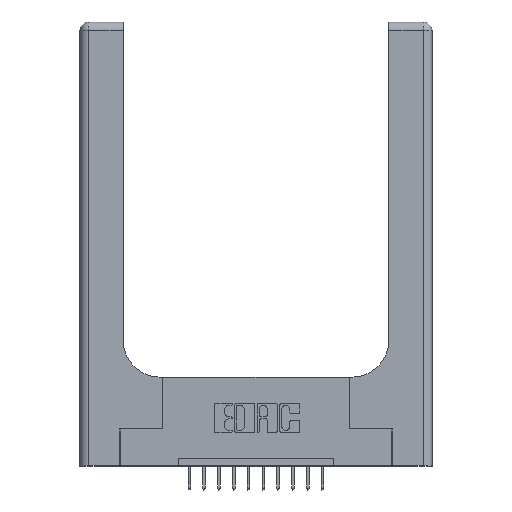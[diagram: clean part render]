
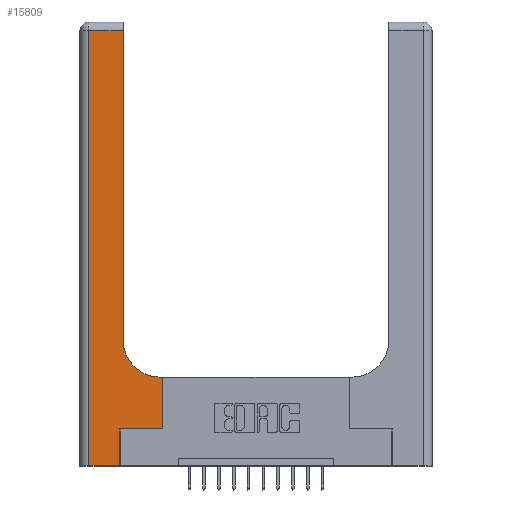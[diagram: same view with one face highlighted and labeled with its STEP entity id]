
A CAD part, top view. The second image highlights one B-rep face of the part: STEP entity #15809.
In plain terms, the highlighted planar face has unit normal (0, 0, 1).
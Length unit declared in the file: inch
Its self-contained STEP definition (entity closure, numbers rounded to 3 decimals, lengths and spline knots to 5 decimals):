
#538 = EDGE_CURVE ( 'NONE', #6167, #1486, #4916, .T. ) ;
#605 = CARTESIAN_POINT ( 'NONE',  ( 0.5585, 0.25, 0.37 ) ) ;
#1486 = VERTEX_POINT ( 'NONE', #4777 ) ;
#1551 = CARTESIAN_POINT ( 'NONE',  ( 0.2915, 0.85, 0.37 ) ) ;
#1597 = LINE ( 'NONE', #6322, #7417 ) ;
#1854 = CARTESIAN_POINT ( 'NONE',  ( 0.2915, 2.94, 0.37 ) ) ;
#2332 = ORIENTED_EDGE ( 'NONE', *, *, #2520, .T. ) ;
#2349 = EDGE_CURVE ( 'NONE', #9811, #10338, #3367, .T. ) ;
#2389 = AXIS2_PLACEMENT_3D ( 'NONE', #6946, #14669, #8240 ) ;
#2520 = EDGE_CURVE ( 'NONE', #7025, #6167, #9157, .T. ) ;
#2974 = LINE ( 'NONE', #16132, #4400 ) ;
#3108 = DIRECTION ( 'NONE',  ( 0., 1., 0. ) ) ;
#3366 = LINE ( 'NONE', #6575, #16765 ) ;
#3367 = LINE ( 'NONE', #4413, #13280 ) ;
#3517 = DIRECTION ( 'NONE',  ( -1., 0., 0. ) ) ;
#3970 = ORIENTED_EDGE ( 'NONE', *, *, #5538, .T. ) ;
#4192 = DIRECTION ( 'NONE',  ( 0., 1., 0. ) ) ;
#4400 = VECTOR ( 'NONE', #16188, 39.37008 ) ;
#4413 = CARTESIAN_POINT ( 'NONE',  ( 0.2915, 3., 0.37 ) ) ;
#4546 = EDGE_LOOP ( 'NONE', ( #6118, #3970, #15986, #16181, #9158, #2332, #13299, #15237, #9519 ) ) ;
#4726 = VECTOR ( 'NONE', #15350, 39.37008 ) ;
#4777 = CARTESIAN_POINT ( 'NONE',  ( 0.5585, 0.6, 0.37 ) ) ;
#4916 = LINE ( 'NONE', #605, #13370 ) ;
#5512 = EDGE_CURVE ( 'NONE', #9137, #9407, #1597, .T. ) ;
#5538 = EDGE_CURVE ( 'NONE', #10338, #9137, #14450, .T. ) ;
#5542 = EDGE_CURVE ( 'NONE', #9407, #9881, #10517, .T. ) ;
#6049 = DIRECTION ( 'NONE',  ( 1., 0., 0. ) ) ;
#6118 = ORIENTED_EDGE ( 'NONE', *, *, #2349, .T. ) ;
#6156 = DIRECTION ( 'NONE',  ( 0., -1., 0. ) ) ;
#6167 = VERTEX_POINT ( 'NONE', #15529 ) ;
#6322 = CARTESIAN_POINT ( 'NONE',  ( 0.06, 3., 0.37 ) ) ;
#6575 = CARTESIAN_POINT ( 'NONE',  ( 0.2915, 0.6, 0.37 ) ) ;
#6946 = CARTESIAN_POINT ( 'NONE',  ( 0.5415, 0.85, 0.37 ) ) ;
#7025 = VERTEX_POINT ( 'NONE', #7530 ) ;
#7233 = FACE_OUTER_BOUND ( 'NONE', #4546, .T. ) ;
#7417 = VECTOR ( 'NONE', #6156, 39.37008 ) ;
#7530 = CARTESIAN_POINT ( 'NONE',  ( 0.269, 0.25, 0.37 ) ) ;
#7691 = PLANE ( 'NONE',  #13101 ) ;
#7851 = CIRCLE ( 'NONE', #2389, 0.25 ) ;
#8240 = DIRECTION ( 'NONE',  ( 1., 0., 0. ) ) ;
#8334 = CARTESIAN_POINT ( 'NONE',  ( 0.5415, 0.6, 0.37 ) ) ;
#9137 = VERTEX_POINT ( 'NONE', #13842 ) ;
#9157 = LINE ( 'NONE', #9891, #13919 ) ;
#9158 = ORIENTED_EDGE ( 'NONE', *, *, #15093, .T. ) ;
#9407 = VERTEX_POINT ( 'NONE', #12059 ) ;
#9519 = ORIENTED_EDGE ( 'NONE', *, *, #16583, .T. ) ;
#9811 = VERTEX_POINT ( 'NONE', #1551 ) ;
#9881 = VERTEX_POINT ( 'NONE', #11748 ) ;
#9891 = CARTESIAN_POINT ( 'NONE',  ( 0.269, 0.25, 0.37 ) ) ;
#10092 = VECTOR ( 'NONE', #12960, 39.37008 ) ;
#10139 = DIRECTION ( 'NONE',  ( 0., 0., -1. ) ) ;
#10338 = VERTEX_POINT ( 'NONE', #1854 ) ;
#10517 = LINE ( 'NONE', #15408, #4726 ) ;
#11688 = EDGE_CURVE ( 'NONE', #1486, #14406, #3366, .T. ) ;
#11748 = CARTESIAN_POINT ( 'NONE',  ( 0.269, 0., 0.37 ) ) ;
#12059 = CARTESIAN_POINT ( 'NONE',  ( 0.06, 0., 0.37 ) ) ;
#12681 = CARTESIAN_POINT ( 'NONE',  ( 0., 3., 0.37 ) ) ;
#12960 = DIRECTION ( 'NONE',  ( -1., 0., 0. ) ) ;
#13101 = AXIS2_PLACEMENT_3D ( 'NONE', #12681, #10139, #3517 ) ;
#13280 = VECTOR ( 'NONE', #4192, 39.37008 ) ;
#13299 = ORIENTED_EDGE ( 'NONE', *, *, #538, .T. ) ;
#13370 = VECTOR ( 'NONE', #3108, 39.37008 ) ;
#13842 = CARTESIAN_POINT ( 'NONE',  ( 0.06, 2.94, 0.37 ) ) ;
#13919 = VECTOR ( 'NONE', #6049, 39.37008 ) ;
#14276 = DIRECTION ( 'NONE',  ( -1., 0., 0. ) ) ;
#14406 = VERTEX_POINT ( 'NONE', #8334 ) ;
#14450 = LINE ( 'NONE', #16846, #10092 ) ;
#14669 = DIRECTION ( 'NONE',  ( 0., 0., -1. ) ) ;
#15093 = EDGE_CURVE ( 'NONE', #9881, #7025, #2974, .T. ) ;
#15237 = ORIENTED_EDGE ( 'NONE', *, *, #11688, .T. ) ;
#15350 = DIRECTION ( 'NONE',  ( 1., 0., 0. ) ) ;
#15408 = CARTESIAN_POINT ( 'NONE',  ( 0., 0., 0.37 ) ) ;
#15529 = CARTESIAN_POINT ( 'NONE',  ( 0.5585, 0.25, 0.37 ) ) ;
#15809 = ADVANCED_FACE ( 'NONE', ( #7233 ), #7691, .F. ) ;
#15986 = ORIENTED_EDGE ( 'NONE', *, *, #5512, .T. ) ;
#16132 = CARTESIAN_POINT ( 'NONE',  ( 0.269, 0., 0.37 ) ) ;
#16181 = ORIENTED_EDGE ( 'NONE', *, *, #5542, .T. ) ;
#16188 = DIRECTION ( 'NONE',  ( 0., 1., 0. ) ) ;
#16583 = EDGE_CURVE ( 'NONE', #14406, #9811, #7851, .T. ) ;
#16765 = VECTOR ( 'NONE', #14276, 39.37008 ) ;
#16846 = CARTESIAN_POINT ( 'NONE',  ( 0., 2.94, 0.37 ) ) ;
